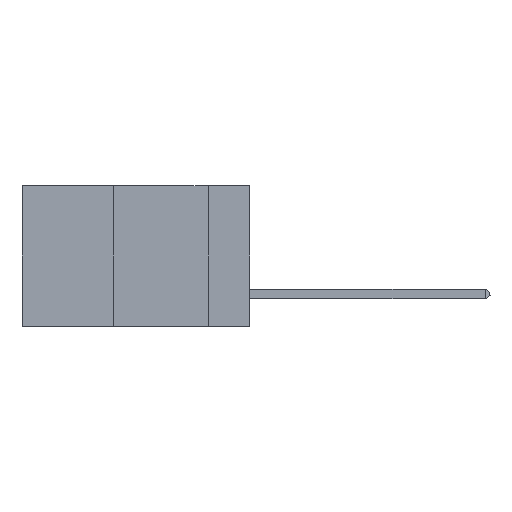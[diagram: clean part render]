
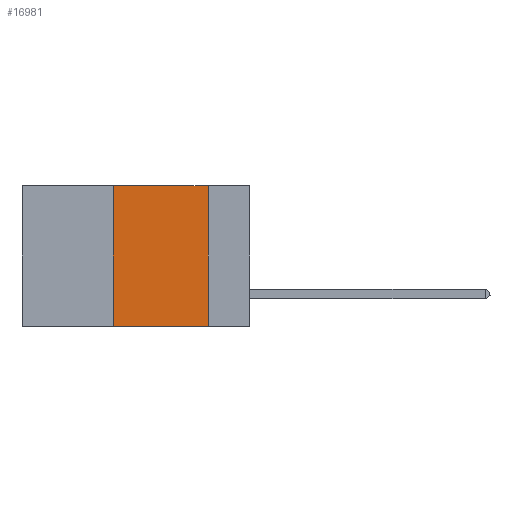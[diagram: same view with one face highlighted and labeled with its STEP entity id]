
A CAD part, left-side view. The second image highlights one B-rep face of the part: STEP entity #16981.
In plain terms, the highlighted planar face has unit normal (-1, 0, 0).
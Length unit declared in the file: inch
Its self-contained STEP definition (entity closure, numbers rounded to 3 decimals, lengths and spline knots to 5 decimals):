
#759 = CARTESIAN_POINT ( 'NONE',  ( 0., 0.6, 0. ) ) ;
#1623 = CARTESIAN_POINT ( 'NONE',  ( 0., 0.11, -0.37 ) ) ;
#3881 = ORIENTED_EDGE ( 'NONE', *, *, #18784, .T. ) ;
#3967 = VERTEX_POINT ( 'NONE', #23390 ) ;
#4037 = VERTEX_POINT ( 'NONE', #25962 ) ;
#5344 = DIRECTION ( 'NONE',  ( 0., 0., 1. ) ) ;
#5574 = VERTEX_POINT ( 'NONE', #1623 ) ;
#5594 = PLANE ( 'NONE',  #20879 ) ;
#6153 = EDGE_CURVE ( 'NONE', #3967, #22844, #11420, .T. ) ;
#6485 = VECTOR ( 'NONE', #15225, 39.37008 ) ;
#7180 = EDGE_CURVE ( 'NONE', #22844, #4037, #23200, .T. ) ;
#8905 = CARTESIAN_POINT ( 'NONE',  ( 0., 0.6, 0. ) ) ;
#9006 = DIRECTION ( 'NONE',  ( 0., -1., 0. ) ) ;
#11420 = LINE ( 'NONE', #24773, #11799 ) ;
#11799 = VECTOR ( 'NONE', #5344, 39.37008 ) ;
#15225 = DIRECTION ( 'NONE',  ( 0., 0., -1. ) ) ;
#15364 = DIRECTION ( 'NONE',  ( 1., 0., 0. ) ) ;
#15526 = DIRECTION ( 'NONE',  ( 0., -1., 0. ) ) ;
#15618 = FACE_OUTER_BOUND ( 'NONE', #24002, .T. ) ;
#16051 = ORIENTED_EDGE ( 'NONE', *, *, #7180, .F. ) ;
#16981 = ADVANCED_FACE ( 'NONE', ( #15618 ), #5594, .F. ) ;
#17584 = CARTESIAN_POINT ( 'NONE',  ( 0., 0.11, 0. ) ) ;
#18784 = EDGE_CURVE ( 'NONE', #3967, #5574, #30465, .T. ) ;
#20879 = AXIS2_PLACEMENT_3D ( 'NONE', #759, #15364, #30244 ) ;
#21202 = ORIENTED_EDGE ( 'NONE', *, *, #25658, .F. ) ;
#21255 = VECTOR ( 'NONE', #9006, 39.37008 ) ;
#22844 = VERTEX_POINT ( 'NONE', #22857 ) ;
#22857 = CARTESIAN_POINT ( 'NONE',  ( 0., 0.36, 0. ) ) ;
#23200 = LINE ( 'NONE', #8905, #21255 ) ;
#23390 = CARTESIAN_POINT ( 'NONE',  ( 0., 0.36, -0.37 ) ) ;
#23963 = VECTOR ( 'NONE', #15526, 39.37008 ) ;
#24002 = EDGE_LOOP ( 'NONE', ( #21202, #16051, #29363, #3881 ) ) ;
#24773 = CARTESIAN_POINT ( 'NONE',  ( 0., 0.36, 0. ) ) ;
#25658 = EDGE_CURVE ( 'NONE', #4037, #5574, #27605, .T. ) ;
#25962 = CARTESIAN_POINT ( 'NONE',  ( 0., 0.11, 0. ) ) ;
#27548 = CARTESIAN_POINT ( 'NONE',  ( 0., 0.6, -0.37 ) ) ;
#27605 = LINE ( 'NONE', #17584, #6485 ) ;
#29363 = ORIENTED_EDGE ( 'NONE', *, *, #6153, .F. ) ;
#30244 = DIRECTION ( 'NONE',  ( 0., 0., -1. ) ) ;
#30465 = LINE ( 'NONE', #27548, #23963 ) ;
